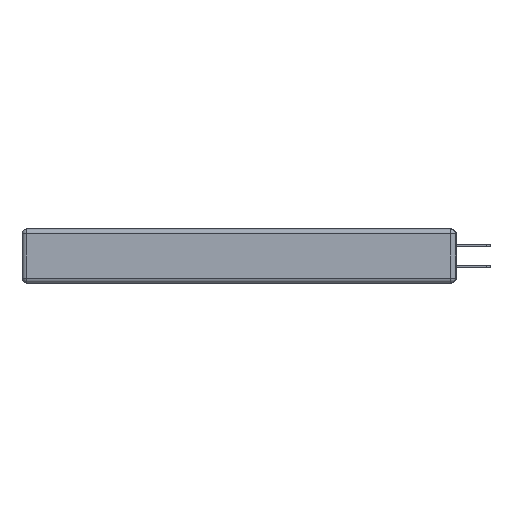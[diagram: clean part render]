
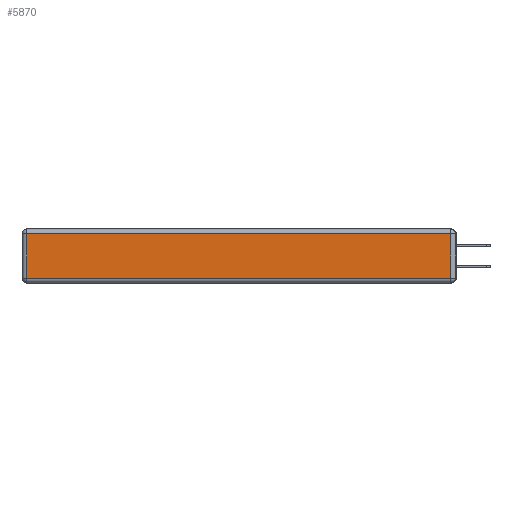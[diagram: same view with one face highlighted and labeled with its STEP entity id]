
A CAD part, left-side view. The second image highlights one B-rep face of the part: STEP entity #5870.
In plain terms, the highlighted planar face has unit normal (-1, 0, 0).
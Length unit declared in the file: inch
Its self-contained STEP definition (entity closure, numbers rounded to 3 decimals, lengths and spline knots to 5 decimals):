
#454 = LINE ( 'NONE', #24357, #18009 ) ;
#472 = AXIS2_PLACEMENT_3D ( 'NONE', #3956, #5795, #12140 ) ;
#2096 = CARTESIAN_POINT ( 'NONE',  ( 0., 0., -0.313 ) ) ;
#3430 = EDGE_CURVE ( 'NONE', #16670, #12899, #454, .T. ) ;
#3956 = CARTESIAN_POINT ( 'NONE',  ( 0., 0., -0.343 ) ) ;
#4104 = LINE ( 'NONE', #12717, #10094 ) ;
#4189 = VERTEX_POINT ( 'NONE', #11051 ) ;
#4452 = DIRECTION ( 'NONE',  ( 0., 1., 0. ) ) ;
#4475 = LINE ( 'NONE', #2096, #12976 ) ;
#5795 = DIRECTION ( 'NONE',  ( -1., 0., 0. ) ) ;
#5870 = ADVANCED_FACE ( 'NONE', ( #24956 ), #19923, .T. ) ;
#6842 = VERTEX_POINT ( 'NONE', #16214 ) ;
#6962 = EDGE_CURVE ( 'NONE', #12899, #6842, #4104, .T. ) ;
#10094 = VECTOR ( 'NONE', #4452, 39.37008 ) ;
#10262 = DIRECTION ( 'NONE',  ( 0., -1., 0. ) ) ;
#11051 = CARTESIAN_POINT ( 'NONE',  ( 0., 2.72, -0.313 ) ) ;
#12140 = DIRECTION ( 'NONE',  ( 0., 0., 1. ) ) ;
#12717 = CARTESIAN_POINT ( 'NONE',  ( 0., 2.75, -0.03 ) ) ;
#12899 = VERTEX_POINT ( 'NONE', #18718 ) ;
#12976 = VECTOR ( 'NONE', #10262, 39.37008 ) ;
#13106 = EDGE_LOOP ( 'NONE', ( #14737, #25255, #21349, #19891 ) ) ;
#13496 = CARTESIAN_POINT ( 'NONE',  ( 0., 2.72, -0.343 ) ) ;
#14737 = ORIENTED_EDGE ( 'NONE', *, *, #22007, .T. ) ;
#15578 = DIRECTION ( 'NONE',  ( 0., 0., -1. ) ) ;
#15948 = LINE ( 'NONE', #13496, #25434 ) ;
#16214 = CARTESIAN_POINT ( 'NONE',  ( 0., 2.72, -0.03 ) ) ;
#16670 = VERTEX_POINT ( 'NONE', #20410 ) ;
#18009 = VECTOR ( 'NONE', #18434, 39.37008 ) ;
#18434 = DIRECTION ( 'NONE',  ( 0., 0., 1. ) ) ;
#18718 = CARTESIAN_POINT ( 'NONE',  ( 0., 0.03, -0.03 ) ) ;
#19891 = ORIENTED_EDGE ( 'NONE', *, *, #25108, .T. ) ;
#19923 = PLANE ( 'NONE',  #472 ) ;
#20410 = CARTESIAN_POINT ( 'NONE',  ( 0., 0.03, -0.313 ) ) ;
#21349 = ORIENTED_EDGE ( 'NONE', *, *, #6962, .T. ) ;
#22007 = EDGE_CURVE ( 'NONE', #4189, #16670, #4475, .T. ) ;
#24357 = CARTESIAN_POINT ( 'NONE',  ( 0., 0.03, -0.343 ) ) ;
#24956 = FACE_OUTER_BOUND ( 'NONE', #13106, .T. ) ;
#25108 = EDGE_CURVE ( 'NONE', #6842, #4189, #15948, .T. ) ;
#25255 = ORIENTED_EDGE ( 'NONE', *, *, #3430, .T. ) ;
#25434 = VECTOR ( 'NONE', #15578, 39.37008 ) ;
